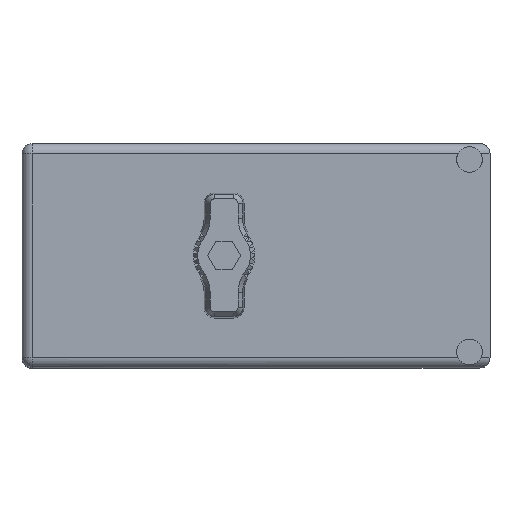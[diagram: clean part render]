
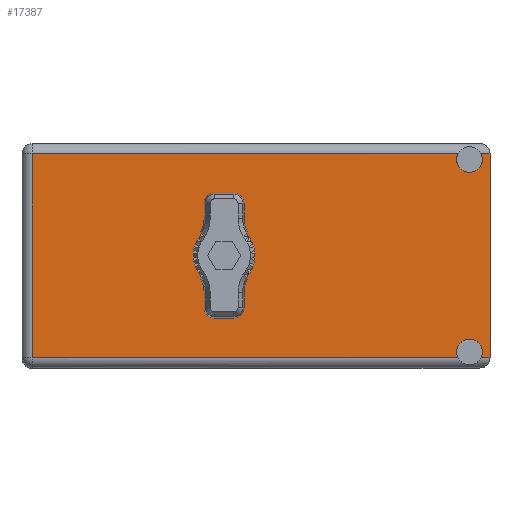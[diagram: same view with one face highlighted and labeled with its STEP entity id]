
A CAD part, top view. The second image highlights one B-rep face of the part: STEP entity #17387.
In plain terms, the highlighted face is planar.
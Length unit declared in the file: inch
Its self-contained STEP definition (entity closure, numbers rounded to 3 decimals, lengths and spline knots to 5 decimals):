
#108 = CARTESIAN_POINT ( 'NONE',  ( 1.59417, 1.93, -0.695 ) ) ;
#489 = CARTESIAN_POINT ( 'NONE',  ( 0., 1.93, 0.17 ) ) ;
#978 = VECTOR ( 'NONE', #22777, 39.37008 ) ;
#4139 = EDGE_CURVE ( 'NONE', #33022, #11706, #94360, .T. ) ;
#6332 = LINE ( 'NONE', #70896, #38682 ) ;
#6702 = CARTESIAN_POINT ( 'NONE',  ( 0., 1.93, 0. ) ) ;
#9411 = CARTESIAN_POINT ( 'NONE',  ( 1.6725, 1.93, -0.656 ) ) ;
#9456 = CARTESIAN_POINT ( 'NONE',  ( 1.6725, 1.93, 0.656 ) ) ;
#10901 = EDGE_LOOP ( 'NONE', ( #45006, #31151, #69260, #68888, #47578, #84492, #79011, #26995, #21441, #23922 ) ) ;
#10984 = PLANE ( 'NONE',  #42510 ) ;
#11706 = VERTEX_POINT ( 'NONE', #65363 ) ;
#14439 = CIRCLE ( 'NONE', #92395, 0.0875 ) ;
#14509 = DIRECTION ( 'NONE',  ( 0., 1., 0. ) ) ;
#15392 = CIRCLE ( 'NONE', #41798, 0.0875 ) ;
#15897 = EDGE_CURVE ( 'NONE', #65261, #86188, #15392, .T. ) ;
#16116 = EDGE_CURVE ( 'NONE', #16548, #53373, #50273, .T. ) ;
#16548 = VERTEX_POINT ( 'NONE', #59590 ) ;
#17387 = ADVANCED_FACE ( 'NONE', ( #97800, #30884 ), #10984, .T. ) ;
#18669 = DIRECTION ( 'NONE',  ( -1., 0., 0. ) ) ;
#21441 = ORIENTED_EDGE ( 'NONE', *, *, #25772, .T. ) ;
#21545 = CARTESIAN_POINT ( 'NONE',  ( -1.3775, 1.93, -0.695 ) ) ;
#22777 = DIRECTION ( 'NONE',  ( 1., 0., 0. ) ) ;
#23767 = CARTESIAN_POINT ( 'NONE',  ( -1.3075, 1.93, -0.765 ) ) ;
#23804 = DIRECTION ( 'NONE',  ( 0., 1., 0. ) ) ;
#23922 = ORIENTED_EDGE ( 'NONE', *, *, #81421, .T. ) ;
#24432 = CARTESIAN_POINT ( 'NONE',  ( 1.8125, 1.93, -0.695 ) ) ;
#24819 = CIRCLE ( 'NONE', #75746, 0.0875 ) ;
#25772 = EDGE_CURVE ( 'NONE', #76116, #86985, #6332, .T. ) ;
#25947 = CARTESIAN_POINT ( 'NONE',  ( 1.8125, 1.93, 0.765 ) ) ;
#26875 = DIRECTION ( 'NONE',  ( 0., 1., 0. ) ) ;
#26995 = ORIENTED_EDGE ( 'NONE', *, *, #47489, .F. ) ;
#28311 = EDGE_LOOP ( 'NONE', ( #52514, #86013 ) ) ;
#29445 = CARTESIAN_POINT ( 'NONE',  ( -1.3075, 1.93, -0.695 ) ) ;
#30884 = FACE_OUTER_BOUND ( 'NONE', #10901, .T. ) ;
#31133 = CIRCLE ( 'NONE', #61084, 0.17 ) ;
#31151 = ORIENTED_EDGE ( 'NONE', *, *, #47246, .F. ) ;
#32462 = DIRECTION ( 'NONE',  ( -1., 0., 0. ) ) ;
#33022 = VERTEX_POINT ( 'NONE', #50931 ) ;
#35452 = AXIS2_PLACEMENT_3D ( 'NONE', #72784, #26875, #49998 ) ;
#37044 = VECTOR ( 'NONE', #70840, 39.37008 ) ;
#37561 = CARTESIAN_POINT ( 'NONE',  ( 1.8125, 1.93, 0.695 ) ) ;
#38107 = EDGE_CURVE ( 'NONE', #61200, #86188, #48599, .T. ) ;
#38682 = VECTOR ( 'NONE', #32462, 39.37008 ) ;
#40174 = LINE ( 'NONE', #23767, #83338 ) ;
#41798 = AXIS2_PLACEMENT_3D ( 'NONE', #9411, #23804, #48284 ) ;
#42007 = VERTEX_POINT ( 'NONE', #78683 ) ;
#42510 = AXIS2_PLACEMENT_3D ( 'NONE', #64498, #87609, #18669 ) ;
#43736 = VECTOR ( 'NONE', #74125, 39.37008 ) ;
#44404 = VERTEX_POINT ( 'NONE', #45363 ) ;
#45006 = ORIENTED_EDGE ( 'NONE', *, *, #4139, .T. ) ;
#45363 = CARTESIAN_POINT ( 'NONE',  ( 1.8125, 1.93, 0.695 ) ) ;
#45568 = CARTESIAN_POINT ( 'NONE',  ( 1.75083, 1.93, -0.695 ) ) ;
#47246 = EDGE_CURVE ( 'NONE', #82680, #11706, #14439, .T. ) ;
#47489 = EDGE_CURVE ( 'NONE', #76116, #65261, #83763, .T. ) ;
#47578 = ORIENTED_EDGE ( 'NONE', *, *, #63211, .F. ) ;
#47662 = EDGE_CURVE ( 'NONE', #53373, #16548, #31133, .T. ) ;
#48284 = DIRECTION ( 'NONE',  ( 0., 0., 1. ) ) ;
#48599 = LINE ( 'NONE', #21545, #43736 ) ;
#49998 = DIRECTION ( 'NONE',  ( 0., 0., 1. ) ) ;
#50273 = CIRCLE ( 'NONE', #55307, 0.17 ) ;
#50931 = CARTESIAN_POINT ( 'NONE',  ( -1.3075, 1.93, 0.695 ) ) ;
#52514 = ORIENTED_EDGE ( 'NONE', *, *, #47662, .F. ) ;
#53373 = VERTEX_POINT ( 'NONE', #489 ) ;
#55307 = AXIS2_PLACEMENT_3D ( 'NONE', #6702, #83364, #75668 ) ;
#59590 = CARTESIAN_POINT ( 'NONE',  ( 0., 1.93, -0.17 ) ) ;
#61084 = AXIS2_PLACEMENT_3D ( 'NONE', #84427, #14509, #83761 ) ;
#61200 = VERTEX_POINT ( 'NONE', #24432 ) ;
#61947 = DIRECTION ( 'NONE',  ( 0., 0., 1. ) ) ;
#63211 = EDGE_CURVE ( 'NONE', #61200, #44404, #79992, .T. ) ;
#63808 = DIRECTION ( 'NONE',  ( 0., 0., 1. ) ) ;
#64498 = CARTESIAN_POINT ( 'NONE',  ( -1.3775, 1.93, -0.765 ) ) ;
#65261 = VERTEX_POINT ( 'NONE', #85398 ) ;
#65363 = CARTESIAN_POINT ( 'NONE',  ( 1.59417, 1.93, 0.695 ) ) ;
#68440 = DIRECTION ( 'NONE',  ( 0., 1., 0. ) ) ;
#68888 = ORIENTED_EDGE ( 'NONE', *, *, #73984, .T. ) ;
#69260 = ORIENTED_EDGE ( 'NONE', *, *, #92025, .F. ) ;
#69727 = DIRECTION ( 'NONE',  ( 0., 1., 0. ) ) ;
#70840 = DIRECTION ( 'NONE',  ( 1., 0., 0. ) ) ;
#70896 = CARTESIAN_POINT ( 'NONE',  ( -1.3775, 1.93, -0.695 ) ) ;
#72784 = CARTESIAN_POINT ( 'NONE',  ( 1.6725, 1.93, -0.656 ) ) ;
#73984 = EDGE_CURVE ( 'NONE', #42007, #44404, #87336, .T. ) ;
#74125 = DIRECTION ( 'NONE',  ( -1., 0., 0. ) ) ;
#75668 = DIRECTION ( 'NONE',  ( 0., 0., 1. ) ) ;
#75746 = AXIS2_PLACEMENT_3D ( 'NONE', #9456, #69727, #77474 ) ;
#76116 = VERTEX_POINT ( 'NONE', #108 ) ;
#77474 = DIRECTION ( 'NONE',  ( 0., 0., 1. ) ) ;
#78683 = CARTESIAN_POINT ( 'NONE',  ( 1.75083, 1.93, 0.695 ) ) ;
#79011 = ORIENTED_EDGE ( 'NONE', *, *, #15897, .F. ) ;
#79992 = LINE ( 'NONE', #25947, #88313 ) ;
#80922 = CARTESIAN_POINT ( 'NONE',  ( 1.6725, 1.93, 0.5685 ) ) ;
#81421 = EDGE_CURVE ( 'NONE', #86985, #33022, #40174, .T. ) ;
#82680 = VERTEX_POINT ( 'NONE', #80922 ) ;
#82903 = DIRECTION ( 'NONE',  ( 0., 0., 1. ) ) ;
#83338 = VECTOR ( 'NONE', #61947, 39.37008 ) ;
#83364 = DIRECTION ( 'NONE',  ( 0., 1., 0. ) ) ;
#83761 = DIRECTION ( 'NONE',  ( 0., 0., 1. ) ) ;
#83763 = CIRCLE ( 'NONE', #35452, 0.0875 ) ;
#84427 = CARTESIAN_POINT ( 'NONE',  ( 0., 1.93, 0. ) ) ;
#84492 = ORIENTED_EDGE ( 'NONE', *, *, #38107, .T. ) ;
#85398 = CARTESIAN_POINT ( 'NONE',  ( 1.6725, 1.93, -0.5685 ) ) ;
#86013 = ORIENTED_EDGE ( 'NONE', *, *, #16116, .F. ) ;
#86188 = VERTEX_POINT ( 'NONE', #45568 ) ;
#86901 = CARTESIAN_POINT ( 'NONE',  ( 1.8125, 1.93, 0.695 ) ) ;
#86985 = VERTEX_POINT ( 'NONE', #29445 ) ;
#87336 = LINE ( 'NONE', #86901, #37044 ) ;
#87609 = DIRECTION ( 'NONE',  ( 0., 1., 0. ) ) ;
#88313 = VECTOR ( 'NONE', #63808, 39.37008 ) ;
#91502 = CARTESIAN_POINT ( 'NONE',  ( 1.6725, 1.93, 0.656 ) ) ;
#92025 = EDGE_CURVE ( 'NONE', #42007, #82680, #24819, .T. ) ;
#92395 = AXIS2_PLACEMENT_3D ( 'NONE', #91502, #68440, #82903 ) ;
#94360 = LINE ( 'NONE', #37561, #978 ) ;
#97800 = FACE_BOUND ( 'NONE', #28311, .T. ) ;
